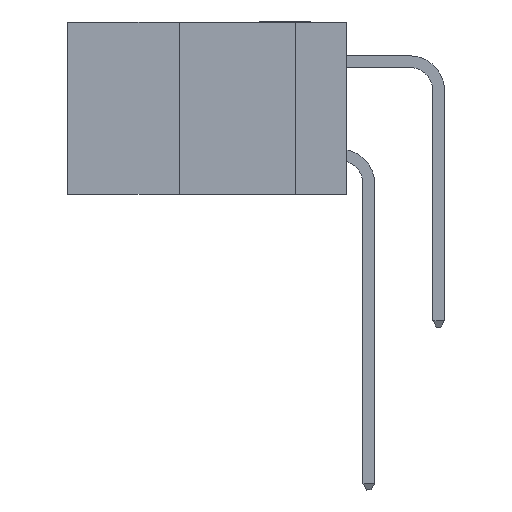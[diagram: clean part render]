
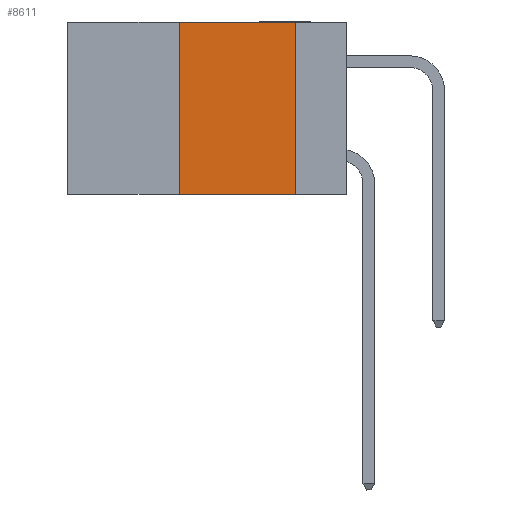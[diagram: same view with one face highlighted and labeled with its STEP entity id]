
A CAD part, left-side view. The second image highlights one B-rep face of the part: STEP entity #8611.
In plain terms, the highlighted planar face has unit normal (-1, 0, 0).
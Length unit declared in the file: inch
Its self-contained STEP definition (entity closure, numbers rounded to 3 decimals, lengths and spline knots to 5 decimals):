
#9 = ORIENTED_EDGE ( 'NONE', *, *, #6058, .F. ) ;
#204 = LINE ( 'NONE', #6940, #8689 ) ;
#402 = DIRECTION ( 'NONE',  ( 1., 0., 0. ) ) ;
#490 = DIRECTION ( 'NONE',  ( 0., -1., 0. ) ) ;
#857 = LINE ( 'NONE', #12164, #11717 ) ;
#1422 = PLANE ( 'NONE',  #11724 ) ;
#1629 = DIRECTION ( 'NONE',  ( 0., 0., 1. ) ) ;
#2610 = CARTESIAN_POINT ( 'NONE',  ( 0., 0.6, 0. ) ) ;
#3611 = ORIENTED_EDGE ( 'NONE', *, *, #12812, .F. ) ;
#3894 = CARTESIAN_POINT ( 'NONE',  ( 0., 0.11, -0.37 ) ) ;
#4667 = EDGE_LOOP ( 'NONE', ( #3611, #8124, #9, #6007 ) ) ;
#5262 = LINE ( 'NONE', #13454, #11300 ) ;
#5563 = CARTESIAN_POINT ( 'NONE',  ( 0., 0.36, 0. ) ) ;
#5941 = FACE_OUTER_BOUND ( 'NONE', #4667, .T. ) ;
#5983 = EDGE_CURVE ( 'NONE', #7154, #8759, #857, .T. ) ;
#6007 = ORIENTED_EDGE ( 'NONE', *, *, #5983, .T. ) ;
#6058 = EDGE_CURVE ( 'NONE', #7154, #13140, #204, .T. ) ;
#6867 = DIRECTION ( 'NONE',  ( 0., -1., 0. ) ) ;
#6940 = CARTESIAN_POINT ( 'NONE',  ( 0., 0.36, 0. ) ) ;
#7154 = VERTEX_POINT ( 'NONE', #11502 ) ;
#7886 = VECTOR ( 'NONE', #8312, 39.37008 ) ;
#7916 = CARTESIAN_POINT ( 'NONE',  ( 0., 0.11, 0. ) ) ;
#7991 = VERTEX_POINT ( 'NONE', #7916 ) ;
#8124 = ORIENTED_EDGE ( 'NONE', *, *, #8721, .F. ) ;
#8312 = DIRECTION ( 'NONE',  ( 0., 0., -1. ) ) ;
#8611 = ADVANCED_FACE ( 'NONE', ( #5941 ), #1422, .F. ) ;
#8689 = VECTOR ( 'NONE', #1629, 39.37008 ) ;
#8721 = EDGE_CURVE ( 'NONE', #13140, #7991, #5262, .T. ) ;
#8759 = VERTEX_POINT ( 'NONE', #3894 ) ;
#9411 = LINE ( 'NONE', #13827, #7886 ) ;
#11300 = VECTOR ( 'NONE', #490, 39.37008 ) ;
#11502 = CARTESIAN_POINT ( 'NONE',  ( 0., 0.36, -0.37 ) ) ;
#11717 = VECTOR ( 'NONE', #6867, 39.37008 ) ;
#11724 = AXIS2_PLACEMENT_3D ( 'NONE', #2610, #402, #12172 ) ;
#12164 = CARTESIAN_POINT ( 'NONE',  ( 0., 0.6, -0.37 ) ) ;
#12172 = DIRECTION ( 'NONE',  ( 0., 0., -1. ) ) ;
#12812 = EDGE_CURVE ( 'NONE', #7991, #8759, #9411, .T. ) ;
#13140 = VERTEX_POINT ( 'NONE', #5563 ) ;
#13454 = CARTESIAN_POINT ( 'NONE',  ( 0., 0.6, 0. ) ) ;
#13827 = CARTESIAN_POINT ( 'NONE',  ( 0., 0.11, 0. ) ) ;
